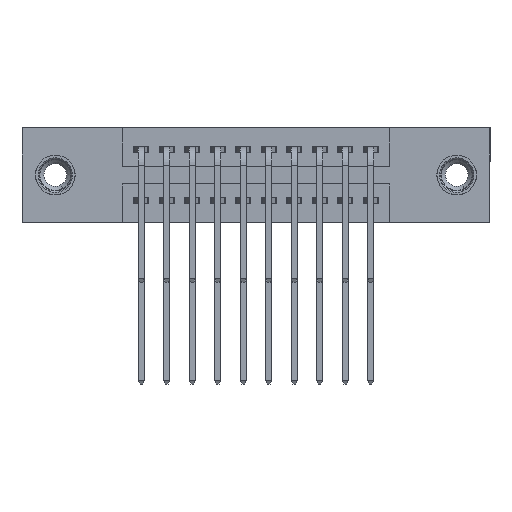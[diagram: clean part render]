
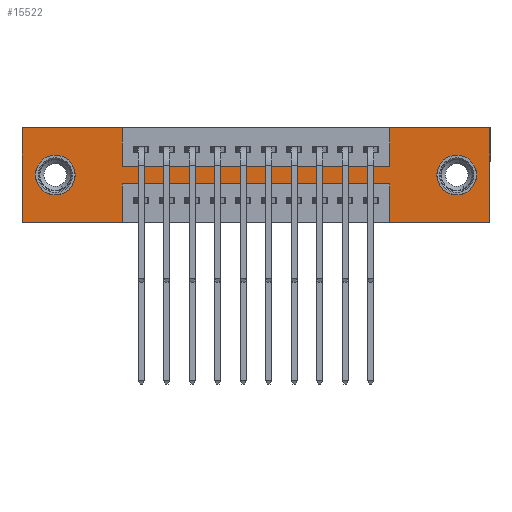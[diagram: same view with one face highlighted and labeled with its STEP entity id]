
A CAD part, front view. The second image highlights one B-rep face of the part: STEP entity #15522.
In plain terms, the highlighted planar face has unit normal (0, -1, 0).
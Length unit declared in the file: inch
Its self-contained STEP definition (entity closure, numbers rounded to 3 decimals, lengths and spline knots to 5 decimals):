
#63 = VERTEX_POINT ( 'NONE', #9010 ) ;
#71 = ORIENTED_EDGE ( 'NONE', *, *, #8186, .T. ) ;
#194 = LINE ( 'NONE', #8679, #7696 ) ;
#339 = CARTESIAN_POINT ( 'NONE',  ( 1.705, 0., -0.185 ) ) ;
#378 = CIRCLE ( 'NONE', #11061, 0.078 ) ;
#762 = LINE ( 'NONE', #11343, #15472 ) ;
#793 = VERTEX_POINT ( 'NONE', #13609 ) ;
#822 = EDGE_LOOP ( 'NONE', ( #7108, #71 ) ) ;
#1046 = AXIS2_PLACEMENT_3D ( 'NONE', #339, #10530, #1970 ) ;
#1118 = LINE ( 'NONE', #2018, #15801 ) ;
#1367 = DIRECTION ( 'NONE',  ( 0., 0., 1. ) ) ;
#1425 = VERTEX_POINT ( 'NONE', #1651 ) ;
#1484 = DIRECTION ( 'NONE',  ( 0., 1., 0. ) ) ;
#1530 = ORIENTED_EDGE ( 'NONE', *, *, #6882, .F. ) ;
#1634 = VERTEX_POINT ( 'NONE', #3641 ) ;
#1651 = CARTESIAN_POINT ( 'NONE',  ( 0.13, 0., -0.107 ) ) ;
#1669 = FACE_OUTER_BOUND ( 'NONE', #3546, .T. ) ;
#1914 = ORIENTED_EDGE ( 'NONE', *, *, #8794, .F. ) ;
#1970 = DIRECTION ( 'NONE',  ( 0., 0., -1. ) ) ;
#2018 = CARTESIAN_POINT ( 'NONE',  ( 0., 0., 0. ) ) ;
#2050 = EDGE_CURVE ( 'NONE', #13821, #1634, #11494, .T. ) ;
#2054 = DIRECTION ( 'NONE',  ( 0., 0., 1. ) ) ;
#2300 = DIRECTION ( 'NONE',  ( 1., 0., 0. ) ) ;
#2438 = CARTESIAN_POINT ( 'NONE',  ( 1.4425, 0., -0.37 ) ) ;
#2934 = LINE ( 'NONE', #10593, #10017 ) ;
#3379 = CARTESIAN_POINT ( 'NONE',  ( 0., 0., -0.37 ) ) ;
#3519 = EDGE_LOOP ( 'NONE', ( #3538, #8279 ) ) ;
#3538 = ORIENTED_EDGE ( 'NONE', *, *, #13420, .T. ) ;
#3546 = EDGE_LOOP ( 'NONE', ( #3930, #5398, #6772, #17515, #6449, #10838, #16727, #1530, #15441, #12709, #1914, #16198 ) ) ;
#3641 = CARTESIAN_POINT ( 'NONE',  ( 1.835, 0., -0.37 ) ) ;
#3868 = DIRECTION ( 'NONE',  ( 1., 0., 0. ) ) ;
#3930 = ORIENTED_EDGE ( 'NONE', *, *, #18112, .F. ) ;
#3931 = CARTESIAN_POINT ( 'NONE',  ( 1.4425, 0., -0.22 ) ) ;
#4185 = CARTESIAN_POINT ( 'NONE',  ( 0.13, 0., -0.185 ) ) ;
#4255 = CARTESIAN_POINT ( 'NONE',  ( 0.3925, 0., -0.22 ) ) ;
#4260 = CARTESIAN_POINT ( 'NONE',  ( 0.3925, 0., -0.37 ) ) ;
#4890 = CARTESIAN_POINT ( 'NONE',  ( 1.4425, 0., -0.15 ) ) ;
#4961 = LINE ( 'NONE', #8100, #11912 ) ;
#4964 = VERTEX_POINT ( 'NONE', #7437 ) ;
#4981 = EDGE_CURVE ( 'NONE', #6367, #1425, #11128, .T. ) ;
#5228 = FACE_BOUND ( 'NONE', #822, .T. ) ;
#5398 = ORIENTED_EDGE ( 'NONE', *, *, #12278, .F. ) ;
#5404 = CARTESIAN_POINT ( 'NONE',  ( 0., 0., -0.37 ) ) ;
#5621 = DIRECTION ( 'NONE',  ( 0., 0., 1. ) ) ;
#5701 = DIRECTION ( 'NONE',  ( 0., 0., -1. ) ) ;
#5793 = CARTESIAN_POINT ( 'NONE',  ( 1.705, 0., -0.263 ) ) ;
#5821 = EDGE_CURVE ( 'NONE', #63, #13821, #6343, .T. ) ;
#5856 = DIRECTION ( 'NONE',  ( -1., 0., 0. ) ) ;
#6193 = DIRECTION ( 'NONE',  ( 0., 0., -1. ) ) ;
#6343 = LINE ( 'NONE', #10824, #16565 ) ;
#6367 = VERTEX_POINT ( 'NONE', #8238 ) ;
#6388 = CARTESIAN_POINT ( 'NONE',  ( 1.835, 0., 0. ) ) ;
#6449 = ORIENTED_EDGE ( 'NONE', *, *, #2050, .F. ) ;
#6678 = DIRECTION ( 'NONE',  ( -1., 0., 0. ) ) ;
#6772 = ORIENTED_EDGE ( 'NONE', *, *, #6778, .F. ) ;
#6778 = EDGE_CURVE ( 'NONE', #15107, #9804, #2934, .T. ) ;
#6882 = EDGE_CURVE ( 'NONE', #793, #13104, #16063, .T. ) ;
#6909 = EDGE_CURVE ( 'NONE', #1634, #15107, #4961, .T. ) ;
#7088 = AXIS2_PLACEMENT_3D ( 'NONE', #3379, #15950, #7673 ) ;
#7108 = ORIENTED_EDGE ( 'NONE', *, *, #18219, .T. ) ;
#7397 = CIRCLE ( 'NONE', #1046, 0.078 ) ;
#7437 = CARTESIAN_POINT ( 'NONE',  ( 1.705, 0., -0.107 ) ) ;
#7661 = AXIS2_PLACEMENT_3D ( 'NONE', #4185, #13936, #5621 ) ;
#7673 = DIRECTION ( 'NONE',  ( 0., 0., -1. ) ) ;
#7696 = VECTOR ( 'NONE', #15600, 39.37008 ) ;
#8100 = CARTESIAN_POINT ( 'NONE',  ( 0., 0., -0.37 ) ) ;
#8186 = EDGE_CURVE ( 'NONE', #16601, #4964, #7397, .T. ) ;
#8198 = VERTEX_POINT ( 'NONE', #9198 ) ;
#8238 = CARTESIAN_POINT ( 'NONE',  ( 0.13, 0., -0.263 ) ) ;
#8279 = ORIENTED_EDGE ( 'NONE', *, *, #4981, .T. ) ;
#8679 = CARTESIAN_POINT ( 'NONE',  ( 0.3925, 0., 0. ) ) ;
#8794 = EDGE_CURVE ( 'NONE', #13789, #10827, #1118, .T. ) ;
#8826 = CIRCLE ( 'NONE', #7661, 0.078 ) ;
#8906 = DIRECTION ( 'NONE',  ( 0., 1., 0. ) ) ;
#9010 = CARTESIAN_POINT ( 'NONE',  ( 1.4425, 0., 0. ) ) ;
#9198 = CARTESIAN_POINT ( 'NONE',  ( 0.3925, 0., -0.37 ) ) ;
#9249 = CARTESIAN_POINT ( 'NONE',  ( 0., 0., -0.37 ) ) ;
#9402 = FACE_BOUND ( 'NONE', #3519, .T. ) ;
#9804 = VERTEX_POINT ( 'NONE', #3931 ) ;
#9923 = VECTOR ( 'NONE', #2300, 39.37008 ) ;
#9981 = VERTEX_POINT ( 'NONE', #18311 ) ;
#10017 = VECTOR ( 'NONE', #2054, 39.37008 ) ;
#10146 = CARTESIAN_POINT ( 'NONE',  ( 1.705, 0., -0.185 ) ) ;
#10326 = LINE ( 'NONE', #12129, #9923 ) ;
#10530 = DIRECTION ( 'NONE',  ( 0., 1., 0. ) ) ;
#10593 = CARTESIAN_POINT ( 'NONE',  ( 1.4425, 0., -0.37 ) ) ;
#10784 = CARTESIAN_POINT ( 'NONE',  ( 0.3925, 0., -0.15 ) ) ;
#10793 = VERTEX_POINT ( 'NONE', #4255 ) ;
#10824 = CARTESIAN_POINT ( 'NONE',  ( 0., 0., 0. ) ) ;
#10827 = VERTEX_POINT ( 'NONE', #18271 ) ;
#10838 = ORIENTED_EDGE ( 'NONE', *, *, #5821, .F. ) ;
#11061 = AXIS2_PLACEMENT_3D ( 'NONE', #10146, #1484, #11500 ) ;
#11128 = CIRCLE ( 'NONE', #14503, 0.078 ) ;
#11343 = CARTESIAN_POINT ( 'NONE',  ( 1.4425, 0., 0. ) ) ;
#11494 = LINE ( 'NONE', #6388, #18497 ) ;
#11500 = DIRECTION ( 'NONE',  ( 0., 0., -1. ) ) ;
#11736 = VECTOR ( 'NONE', #16539, 39.37008 ) ;
#11741 = PLANE ( 'NONE',  #7088 ) ;
#11856 = EDGE_CURVE ( 'NONE', #10827, #9981, #10326, .T. ) ;
#11912 = VECTOR ( 'NONE', #6678, 39.37008 ) ;
#11955 = DIRECTION ( 'NONE',  ( 0., 0., 1. ) ) ;
#12129 = CARTESIAN_POINT ( 'NONE',  ( 0., 0., 0. ) ) ;
#12182 = LINE ( 'NONE', #5404, #11736 ) ;
#12278 = EDGE_CURVE ( 'NONE', #9804, #10793, #14854, .T. ) ;
#12353 = VECTOR ( 'NONE', #13569, 39.37008 ) ;
#12709 = ORIENTED_EDGE ( 'NONE', *, *, #11856, .F. ) ;
#12748 = CARTESIAN_POINT ( 'NONE',  ( 0.3925, 0., -0.22 ) ) ;
#12909 = EDGE_CURVE ( 'NONE', #13104, #63, #762, .T. ) ;
#13104 = VERTEX_POINT ( 'NONE', #4890 ) ;
#13420 = EDGE_CURVE ( 'NONE', #1425, #6367, #8826, .T. ) ;
#13569 = DIRECTION ( 'NONE',  ( 1., 0., 0. ) ) ;
#13609 = CARTESIAN_POINT ( 'NONE',  ( 0.3925, 0., -0.15 ) ) ;
#13789 = VERTEX_POINT ( 'NONE', #9249 ) ;
#13821 = VERTEX_POINT ( 'NONE', #14759 ) ;
#13936 = DIRECTION ( 'NONE',  ( 0., 1., 0. ) ) ;
#14186 = EDGE_CURVE ( 'NONE', #9981, #793, #194, .T. ) ;
#14424 = VECTOR ( 'NONE', #5856, 39.37008 ) ;
#14503 = AXIS2_PLACEMENT_3D ( 'NONE', #17195, #8906, #17731 ) ;
#14536 = VECTOR ( 'NONE', #5701, 39.37008 ) ;
#14759 = CARTESIAN_POINT ( 'NONE',  ( 1.835, 0., 0. ) ) ;
#14854 = LINE ( 'NONE', #12748, #14424 ) ;
#14973 = LINE ( 'NONE', #4260, #14536 ) ;
#15107 = VERTEX_POINT ( 'NONE', #2438 ) ;
#15112 = EDGE_CURVE ( 'NONE', #8198, #13789, #12182, .T. ) ;
#15441 = ORIENTED_EDGE ( 'NONE', *, *, #14186, .F. ) ;
#15472 = VECTOR ( 'NONE', #1367, 39.37008 ) ;
#15522 = ADVANCED_FACE ( 'NONE', ( #5228, #9402, #1669 ), #11741, .T. ) ;
#15600 = DIRECTION ( 'NONE',  ( 0., 0., -1. ) ) ;
#15801 = VECTOR ( 'NONE', #11955, 39.37008 ) ;
#15950 = DIRECTION ( 'NONE',  ( 0., -1., 0. ) ) ;
#16063 = LINE ( 'NONE', #10784, #12353 ) ;
#16198 = ORIENTED_EDGE ( 'NONE', *, *, #15112, .F. ) ;
#16539 = DIRECTION ( 'NONE',  ( -1., 0., 0. ) ) ;
#16565 = VECTOR ( 'NONE', #3868, 39.37008 ) ;
#16601 = VERTEX_POINT ( 'NONE', #5793 ) ;
#16727 = ORIENTED_EDGE ( 'NONE', *, *, #12909, .F. ) ;
#17195 = CARTESIAN_POINT ( 'NONE',  ( 0.13, 0., -0.185 ) ) ;
#17515 = ORIENTED_EDGE ( 'NONE', *, *, #6909, .F. ) ;
#17731 = DIRECTION ( 'NONE',  ( 0., 0., 1. ) ) ;
#18112 = EDGE_CURVE ( 'NONE', #10793, #8198, #14973, .T. ) ;
#18219 = EDGE_CURVE ( 'NONE', #4964, #16601, #378, .T. ) ;
#18271 = CARTESIAN_POINT ( 'NONE',  ( 0., 0., 0. ) ) ;
#18311 = CARTESIAN_POINT ( 'NONE',  ( 0.3925, 0., 0. ) ) ;
#18497 = VECTOR ( 'NONE', #6193, 39.37008 ) ;
